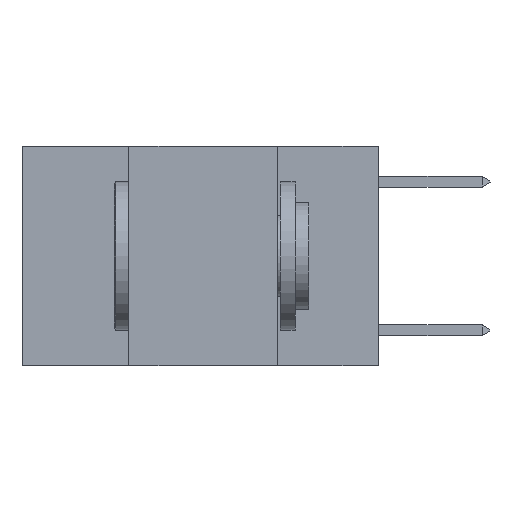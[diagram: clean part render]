
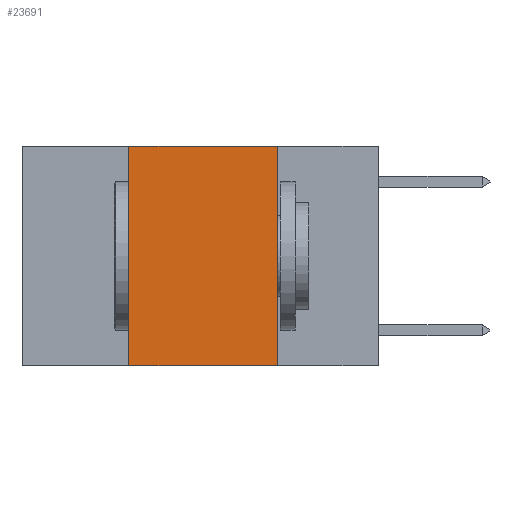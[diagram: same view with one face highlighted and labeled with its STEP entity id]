
A CAD part, left-side view. The second image highlights one B-rep face of the part: STEP entity #23691.
In plain terms, the highlighted planar face has unit normal (-1, 0, 0).
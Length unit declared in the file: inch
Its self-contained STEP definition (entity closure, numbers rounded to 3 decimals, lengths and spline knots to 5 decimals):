
#2763 = VECTOR ( 'NONE', #27412, 39.37008 ) ;
#3801 = EDGE_LOOP ( 'NONE', ( #28662, #15831, #26069, #27554 ) ) ;
#3927 = CARTESIAN_POINT ( 'NONE',  ( 0., 0.6, 0. ) ) ;
#4067 = LINE ( 'NONE', #28637, #30461 ) ;
#4124 = CARTESIAN_POINT ( 'NONE',  ( 0., 0.42, -0.37 ) ) ;
#6283 = DIRECTION ( 'NONE',  ( 0., 0., -1. ) ) ;
#6993 = DIRECTION ( 'NONE',  ( 0., -1., 0. ) ) ;
#8292 = VERTEX_POINT ( 'NONE', #10064 ) ;
#10064 = CARTESIAN_POINT ( 'NONE',  ( 0., 0.17, 0. ) ) ;
#10200 = DIRECTION ( 'NONE',  ( 1., 0., 0. ) ) ;
#10356 = FACE_OUTER_BOUND ( 'NONE', #3801, .T. ) ;
#10412 = EDGE_CURVE ( 'NONE', #20878, #13904, #21101, .T. ) ;
#10665 = DIRECTION ( 'NONE',  ( 0., 0., -1. ) ) ;
#10871 = CARTESIAN_POINT ( 'NONE',  ( 0., 0.17, -0.37 ) ) ;
#12735 = EDGE_CURVE ( 'NONE', #8292, #13904, #4067, .T. ) ;
#13473 = CARTESIAN_POINT ( 'NONE',  ( 0., 0.42, 0. ) ) ;
#13904 = VERTEX_POINT ( 'NONE', #10871 ) ;
#14440 = VERTEX_POINT ( 'NONE', #25125 ) ;
#15598 = CARTESIAN_POINT ( 'NONE',  ( 0., 0.6, 0. ) ) ;
#15831 = ORIENTED_EDGE ( 'NONE', *, *, #28784, .F. ) ;
#17649 = PLANE ( 'NONE',  #29983 ) ;
#20069 = VECTOR ( 'NONE', #30155, 39.37008 ) ;
#20764 = EDGE_CURVE ( 'NONE', #20878, #14440, #30619, .T. ) ;
#20800 = VECTOR ( 'NONE', #6993, 39.37008 ) ;
#20878 = VERTEX_POINT ( 'NONE', #4124 ) ;
#21101 = LINE ( 'NONE', #23507, #20800 ) ;
#23507 = CARTESIAN_POINT ( 'NONE',  ( 0., 0.6, -0.37 ) ) ;
#23691 = ADVANCED_FACE ( 'NONE', ( #10356 ), #17649, .F. ) ;
#25125 = CARTESIAN_POINT ( 'NONE',  ( 0., 0.42, 0. ) ) ;
#25657 = LINE ( 'NONE', #3927, #2763 ) ;
#26069 = ORIENTED_EDGE ( 'NONE', *, *, #20764, .F. ) ;
#27412 = DIRECTION ( 'NONE',  ( 0., -1., 0. ) ) ;
#27554 = ORIENTED_EDGE ( 'NONE', *, *, #10412, .T. ) ;
#28637 = CARTESIAN_POINT ( 'NONE',  ( 0., 0.17, 0. ) ) ;
#28662 = ORIENTED_EDGE ( 'NONE', *, *, #12735, .F. ) ;
#28784 = EDGE_CURVE ( 'NONE', #14440, #8292, #25657, .T. ) ;
#29983 = AXIS2_PLACEMENT_3D ( 'NONE', #15598, #10200, #10665 ) ;
#30155 = DIRECTION ( 'NONE',  ( 0., 0., 1. ) ) ;
#30461 = VECTOR ( 'NONE', #6283, 39.37008 ) ;
#30619 = LINE ( 'NONE', #13473, #20069 ) ;
